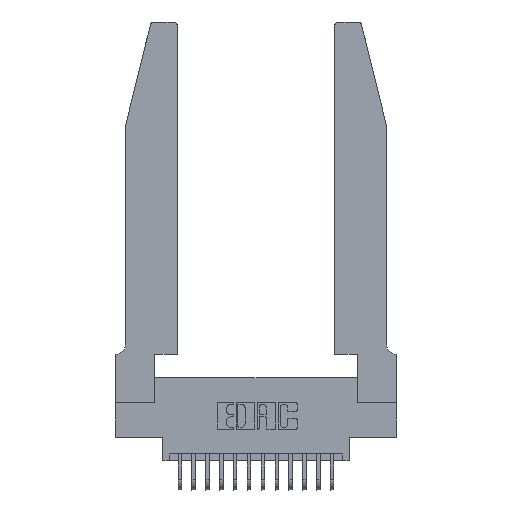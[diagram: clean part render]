
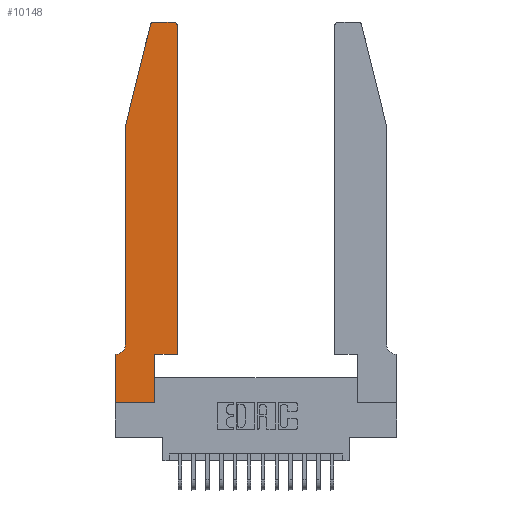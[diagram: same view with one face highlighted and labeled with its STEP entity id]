
A CAD part, top view. The second image highlights one B-rep face of the part: STEP entity #10148.
In plain terms, the highlighted planar face has unit normal (0, 0, 1).
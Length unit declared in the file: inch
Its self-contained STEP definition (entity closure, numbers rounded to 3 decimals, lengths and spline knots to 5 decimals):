
#64 = CIRCLE ( 'NONE', #7551, 0.03 ) ;
#232 = AXIS2_PLACEMENT_3D ( 'NONE', #13164, #13146, #13131 ) ;
#420 = CARTESIAN_POINT ( 'NONE',  ( 0.0055, 0.42, 0.37 ) ) ;
#677 = EDGE_CURVE ( 'NONE', #15984, #13098, #8540, .T. ) ;
#1251 = VERTEX_POINT ( 'NONE', #7507 ) ;
#1471 = VERTEX_POINT ( 'NONE', #6986 ) ;
#1478 = DIRECTION ( 'NONE',  ( 0., -1., 0. ) ) ;
#1490 = EDGE_CURVE ( 'NONE', #6695, #15984, #6294, .T. ) ;
#1766 = CARTESIAN_POINT ( 'NONE',  ( 0.0755, 0.35, 0.37 ) ) ;
#1920 = ORIENTED_EDGE ( 'NONE', *, *, #11172, .T. ) ;
#1950 = VERTEX_POINT ( 'NONE', #9119 ) ;
#1966 = DIRECTION ( 'NONE',  ( -1., 0., 0. ) ) ;
#2037 = VERTEX_POINT ( 'NONE', #12991 ) ;
#2704 = LINE ( 'NONE', #10477, #10558 ) ;
#3157 = CIRCLE ( 'NONE', #11015, 0.07 ) ;
#3193 = DIRECTION ( 'NONE',  ( -0.239, -0.971, 0. ) ) ;
#3262 = CARTESIAN_POINT ( 'NONE',  ( 0.25487, 2.72718, 0.37 ) ) ;
#3311 = EDGE_CURVE ( 'NONE', #1251, #1950, #19261, .T. ) ;
#3727 = ORIENTED_EDGE ( 'NONE', *, *, #6337, .T. ) ;
#3954 = CARTESIAN_POINT ( 'NONE',  ( 0.2865, 0.35, 0.37 ) ) ;
#4014 = CARTESIAN_POINT ( 'NONE',  ( 0.2605, 2.75, 0.37 ) ) ;
#4178 = EDGE_CURVE ( 'NONE', #1471, #16578, #15173, .T. ) ;
#4216 = DIRECTION ( 'NONE',  ( 0., -1., 0. ) ) ;
#4714 = VECTOR ( 'NONE', #18320, 39.37008 ) ;
#4765 = LINE ( 'NONE', #17022, #15269 ) ;
#4777 = VECTOR ( 'NONE', #9612, 39.37008 ) ;
#5581 = DIRECTION ( 'NONE',  ( 0., 0., 1. ) ) ;
#6096 = PLANE ( 'NONE',  #9160 ) ;
#6102 = CARTESIAN_POINT ( 'NONE',  ( 0.284, 2.75, 0.37 ) ) ;
#6294 = LINE ( 'NONE', #4014, #10944 ) ;
#6337 = EDGE_CURVE ( 'NONE', #14770, #6695, #64, .T. ) ;
#6695 = VERTEX_POINT ( 'NONE', #9477 ) ;
#6919 = FACE_OUTER_BOUND ( 'NONE', #15332, .T. ) ;
#6986 = CARTESIAN_POINT ( 'NONE',  ( 0.0055, 0.35, 0.37 ) ) ;
#7507 = CARTESIAN_POINT ( 'NONE',  ( 0., 0., 0.37 ) ) ;
#7551 = AXIS2_PLACEMENT_3D ( 'NONE', #14905, #5581, #16454 ) ;
#7594 = EDGE_CURVE ( 'NONE', #1950, #13483, #12157, .T. ) ;
#7798 = CARTESIAN_POINT ( 'NONE',  ( 0.4505, 2.72, 0.37 ) ) ;
#7919 = CARTESIAN_POINT ( 'NONE',  ( 0.0755, 2., 0.37 ) ) ;
#8247 = ORIENTED_EDGE ( 'NONE', *, *, #1490, .T. ) ;
#8540 = CIRCLE ( 'NONE', #232, 0.03 ) ;
#8759 = VERTEX_POINT ( 'NONE', #9508 ) ;
#8882 = CARTESIAN_POINT ( 'NONE',  ( 0.2865, 0.35, 0.37 ) ) ;
#9098 = CARTESIAN_POINT ( 'NONE',  ( 0., 0., 0.37 ) ) ;
#9119 = CARTESIAN_POINT ( 'NONE',  ( 0.2865, 0., 0.37 ) ) ;
#9160 = AXIS2_PLACEMENT_3D ( 'NONE', #18472, #9247, #20007 ) ;
#9179 = ORIENTED_EDGE ( 'NONE', *, *, #7594, .T. ) ;
#9247 = DIRECTION ( 'NONE',  ( 0., 0., 1. ) ) ;
#9302 = LINE ( 'NONE', #7919, #9797 ) ;
#9477 = CARTESIAN_POINT ( 'NONE',  ( 0.4205, 2.75, 0.37 ) ) ;
#9490 = CARTESIAN_POINT ( 'NONE',  ( 0.4505, 0.35, 0.37 ) ) ;
#9508 = CARTESIAN_POINT ( 'NONE',  ( 0.0755, 0.42, 0.37 ) ) ;
#9612 = DIRECTION ( 'NONE',  ( 1., 0., 0. ) ) ;
#9797 = VECTOR ( 'NONE', #3193, 39.37008 ) ;
#9901 = VERTEX_POINT ( 'NONE', #11111 ) ;
#10148 = ADVANCED_FACE ( 'NONE', ( #6919 ), #6096, .T. ) ;
#10477 = CARTESIAN_POINT ( 'NONE',  ( 0., 0., 0.37 ) ) ;
#10558 = VECTOR ( 'NONE', #4216, 39.37008 ) ;
#10944 = VECTOR ( 'NONE', #11565, 39.37008 ) ;
#11015 = AXIS2_PLACEMENT_3D ( 'NONE', #420, #11303, #1966 ) ;
#11060 = VECTOR ( 'NONE', #17304, 39.37008 ) ;
#11111 = CARTESIAN_POINT ( 'NONE',  ( 0.4505, 0.35, 0.37 ) ) ;
#11172 = EDGE_CURVE ( 'NONE', #16578, #1251, #2704, .T. ) ;
#11200 = ORIENTED_EDGE ( 'NONE', *, *, #677, .T. ) ;
#11248 = ORIENTED_EDGE ( 'NONE', *, *, #13676, .T. ) ;
#11303 = DIRECTION ( 'NONE',  ( 0., 0., -1. ) ) ;
#11430 = EDGE_CURVE ( 'NONE', #13098, #2037, #9302, .T. ) ;
#11565 = DIRECTION ( 'NONE',  ( -1., 0., 0. ) ) ;
#12067 = EDGE_CURVE ( 'NONE', #8759, #1471, #3157, .T. ) ;
#12157 = LINE ( 'NONE', #3954, #19852 ) ;
#12298 = CARTESIAN_POINT ( 'NONE',  ( 0., 0.35, 0.37 ) ) ;
#12299 = ORIENTED_EDGE ( 'NONE', *, *, #16637, .T. ) ;
#12991 = CARTESIAN_POINT ( 'NONE',  ( 0.0755, 2., 0.37 ) ) ;
#13094 = EDGE_CURVE ( 'NONE', #9901, #14770, #14071, .T. ) ;
#13098 = VERTEX_POINT ( 'NONE', #3262 ) ;
#13131 = DIRECTION ( 'NONE',  ( 1., 0., 0. ) ) ;
#13144 = ORIENTED_EDGE ( 'NONE', *, *, #11430, .T. ) ;
#13146 = DIRECTION ( 'NONE',  ( 0., 0., 1. ) ) ;
#13164 = CARTESIAN_POINT ( 'NONE',  ( 0.284, 2.72, 0.37 ) ) ;
#13483 = VERTEX_POINT ( 'NONE', #8882 ) ;
#13570 = VECTOR ( 'NONE', #17191, 39.37008 ) ;
#13676 = EDGE_CURVE ( 'NONE', #13483, #9901, #17190, .T. ) ;
#14071 = LINE ( 'NONE', #9490, #13570 ) ;
#14770 = VERTEX_POINT ( 'NONE', #7798 ) ;
#14905 = CARTESIAN_POINT ( 'NONE',  ( 0.4205, 2.72, 0.37 ) ) ;
#14929 = DIRECTION ( 'NONE',  ( 0., 1., 0. ) ) ;
#15173 = LINE ( 'NONE', #1766, #11060 ) ;
#15269 = VECTOR ( 'NONE', #1478, 39.37008 ) ;
#15332 = EDGE_LOOP ( 'NONE', ( #8247, #11200, #13144, #12299, #16021, #16394, #1920, #17735, #9179, #11248, #15644, #3727 ) ) ;
#15644 = ORIENTED_EDGE ( 'NONE', *, *, #13094, .T. ) ;
#15984 = VERTEX_POINT ( 'NONE', #6102 ) ;
#16021 = ORIENTED_EDGE ( 'NONE', *, *, #12067, .T. ) ;
#16394 = ORIENTED_EDGE ( 'NONE', *, *, #4178, .T. ) ;
#16454 = DIRECTION ( 'NONE',  ( 1., 0., 0. ) ) ;
#16578 = VERTEX_POINT ( 'NONE', #12298 ) ;
#16637 = EDGE_CURVE ( 'NONE', #2037, #8759, #4765, .T. ) ;
#17022 = CARTESIAN_POINT ( 'NONE',  ( 0.0755, 2., 0.37 ) ) ;
#17190 = LINE ( 'NONE', #18757, #4777 ) ;
#17191 = DIRECTION ( 'NONE',  ( 0., 1., 0. ) ) ;
#17304 = DIRECTION ( 'NONE',  ( -1., 0., 0. ) ) ;
#17735 = ORIENTED_EDGE ( 'NONE', *, *, #3311, .T. ) ;
#18320 = DIRECTION ( 'NONE',  ( 1., 0., 0. ) ) ;
#18472 = CARTESIAN_POINT ( 'NONE',  ( 0., 0.35, 0.37 ) ) ;
#18757 = CARTESIAN_POINT ( 'NONE',  ( 0.4505, 0.35, 0.37 ) ) ;
#19261 = LINE ( 'NONE', #9098, #4714 ) ;
#19852 = VECTOR ( 'NONE', #14929, 39.37008 ) ;
#20007 = DIRECTION ( 'NONE',  ( 1., 0., 0. ) ) ;
